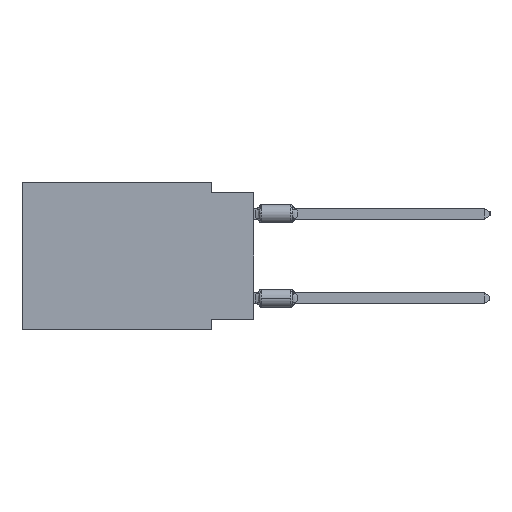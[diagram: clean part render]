
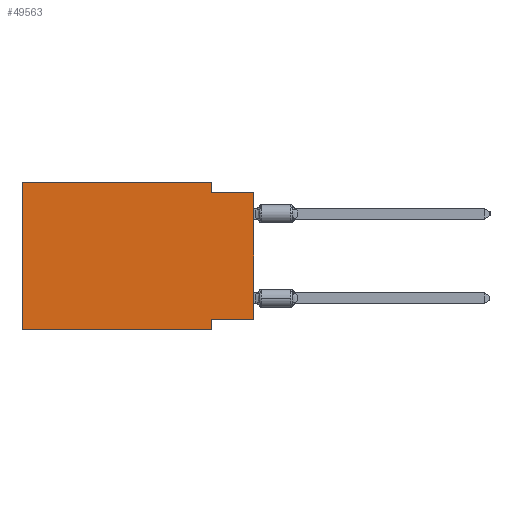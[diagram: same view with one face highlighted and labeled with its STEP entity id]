
A CAD part, left-side view. The second image highlights one B-rep face of the part: STEP entity #49563.
In plain terms, the highlighted planar face has unit normal (-1, 0, 0).
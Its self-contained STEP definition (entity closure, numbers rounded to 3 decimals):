
#13 = CARTESIAN_POINT ( 'NONE',  ( 0., 13.97, -8.89 ) ) ;
#1516 = DIRECTION ( 'NONE',  ( 0., 0., -1. ) ) ;
#2575 = PLANE ( 'NONE',  #17618 ) ;
#2719 = VECTOR ( 'NONE', #50035, 1000. ) ;
#4625 = LINE ( 'NONE', #13, #40065 ) ;
#4858 = CARTESIAN_POINT ( 'NONE',  ( 0., 2.54, 0. ) ) ;
#4893 = ORIENTED_EDGE ( 'NONE', *, *, #26462, .F. ) ;
#5653 = ORIENTED_EDGE ( 'NONE', *, *, #13445, .T. ) ;
#6401 = CARTESIAN_POINT ( 'NONE',  ( 0., 13.97, 0. ) ) ;
#6999 = ORIENTED_EDGE ( 'NONE', *, *, #13804, .F. ) ;
#7385 = ORIENTED_EDGE ( 'NONE', *, *, #47390, .T. ) ;
#9196 = VERTEX_POINT ( 'NONE', #24516 ) ;
#11791 = ORIENTED_EDGE ( 'NONE', *, *, #27098, .F. ) ;
#12167 = CARTESIAN_POINT ( 'NONE',  ( 0., 13.97, 0. ) ) ;
#12422 = DIRECTION ( 'NONE',  ( 0., -1., 0. ) ) ;
#12436 = VERTEX_POINT ( 'NONE', #28757 ) ;
#12577 = LINE ( 'NONE', #28853, #2719 ) ;
#13445 = EDGE_CURVE ( 'NONE', #9196, #48112, #4625, .T. ) ;
#13468 = DIRECTION ( 'NONE',  ( 0., 0., 1. ) ) ;
#13590 = VECTOR ( 'NONE', #21954, 1000. ) ;
#13804 = EDGE_CURVE ( 'NONE', #9196, #12436, #21872, .T. ) ;
#13872 = CARTESIAN_POINT ( 'NONE',  ( 0., 2.54, -8.89 ) ) ;
#14706 = VECTOR ( 'NONE', #44499, 1000. ) ;
#15356 = VERTEX_POINT ( 'NONE', #37390 ) ;
#15758 = ORIENTED_EDGE ( 'NONE', *, *, #45262, .F. ) ;
#17378 = DIRECTION ( 'NONE',  ( 0., -1., 0. ) ) ;
#17618 = AXIS2_PLACEMENT_3D ( 'NONE', #6401, #51195, #1516 ) ;
#18277 = EDGE_CURVE ( 'NONE', #12436, #47455, #20846, .T. ) ;
#18619 = ORIENTED_EDGE ( 'NONE', *, *, #39600, .F. ) ;
#20846 = LINE ( 'NONE', #21651, #39063 ) ;
#21651 = CARTESIAN_POINT ( 'NONE',  ( 0., 13.97, 0. ) ) ;
#21653 = CARTESIAN_POINT ( 'NONE',  ( 0., 0., -8.255 ) ) ;
#21872 = LINE ( 'NONE', #12167, #34072 ) ;
#21954 = DIRECTION ( 'NONE',  ( 0., 0., -1. ) ) ;
#22610 = CARTESIAN_POINT ( 'NONE',  ( 0., 0., -8.255 ) ) ;
#24516 = CARTESIAN_POINT ( 'NONE',  ( 0., 13.97, -8.89 ) ) ;
#24795 = CARTESIAN_POINT ( 'NONE',  ( 0., 2.54, 0. ) ) ;
#25989 = VECTOR ( 'NONE', #42357, 1000. ) ;
#26462 = EDGE_CURVE ( 'NONE', #43614, #38085, #29266, .T. ) ;
#27098 = EDGE_CURVE ( 'NONE', #47455, #38611, #30095, .T. ) ;
#28757 = CARTESIAN_POINT ( 'NONE',  ( 0., 13.97, 0. ) ) ;
#28853 = CARTESIAN_POINT ( 'NONE',  ( 0., 0., 0. ) ) ;
#29266 = LINE ( 'NONE', #21653, #32649 ) ;
#30095 = LINE ( 'NONE', #4858, #13590 ) ;
#31108 = FACE_OUTER_BOUND ( 'NONE', #40357, .T. ) ;
#32649 = VECTOR ( 'NONE', #38206, 1000. ) ;
#33698 = ORIENTED_EDGE ( 'NONE', *, *, #18277, .F. ) ;
#34072 = VECTOR ( 'NONE', #13468, 1000. ) ;
#37390 = CARTESIAN_POINT ( 'NONE',  ( 0., 0., -0.635 ) ) ;
#37977 = CARTESIAN_POINT ( 'NONE',  ( 0., 2.54, -8.255 ) ) ;
#38085 = VERTEX_POINT ( 'NONE', #37977 ) ;
#38206 = DIRECTION ( 'NONE',  ( 0., 1., 0. ) ) ;
#38611 = VERTEX_POINT ( 'NONE', #51979 ) ;
#39063 = VECTOR ( 'NONE', #12422, 1000. ) ;
#39600 = EDGE_CURVE ( 'NONE', #38611, #15356, #41491, .T. ) ;
#40065 = VECTOR ( 'NONE', #17378, 1000. ) ;
#40357 = EDGE_LOOP ( 'NONE', ( #7385, #18619, #11791, #33698, #6999, #5653, #15758, #4893 ) ) ;
#40426 = CARTESIAN_POINT ( 'NONE',  ( 0., 0., -0.635 ) ) ;
#41491 = LINE ( 'NONE', #40426, #14706 ) ;
#42357 = DIRECTION ( 'NONE',  ( 0., 0., -1. ) ) ;
#43183 = LINE ( 'NONE', #13872, #25989 ) ;
#43614 = VERTEX_POINT ( 'NONE', #22610 ) ;
#44499 = DIRECTION ( 'NONE',  ( 0., -1., 0. ) ) ;
#45262 = EDGE_CURVE ( 'NONE', #38085, #48112, #43183, .T. ) ;
#47390 = EDGE_CURVE ( 'NONE', #43614, #15356, #12577, .T. ) ;
#47455 = VERTEX_POINT ( 'NONE', #24795 ) ;
#48112 = VERTEX_POINT ( 'NONE', #53377 ) ;
#49563 = ADVANCED_FACE ( 'NONE', ( #31108 ), #2575, .F. ) ;
#50035 = DIRECTION ( 'NONE',  ( 0., 0., 1. ) ) ;
#51195 = DIRECTION ( 'NONE',  ( 1., 0., 0. ) ) ;
#51979 = CARTESIAN_POINT ( 'NONE',  ( 0., 2.54, -0.635 ) ) ;
#53377 = CARTESIAN_POINT ( 'NONE',  ( 0., 2.54, -8.89 ) ) ;
